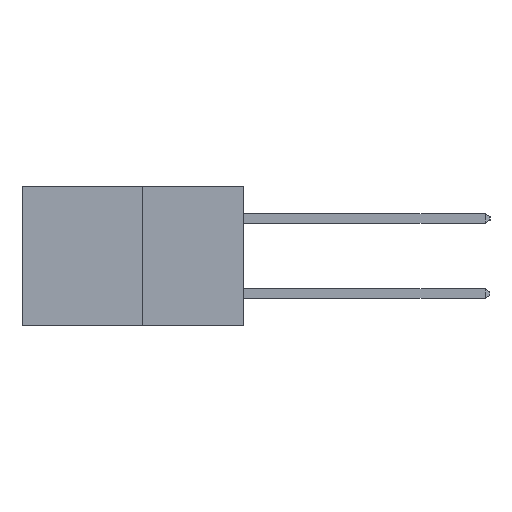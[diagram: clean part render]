
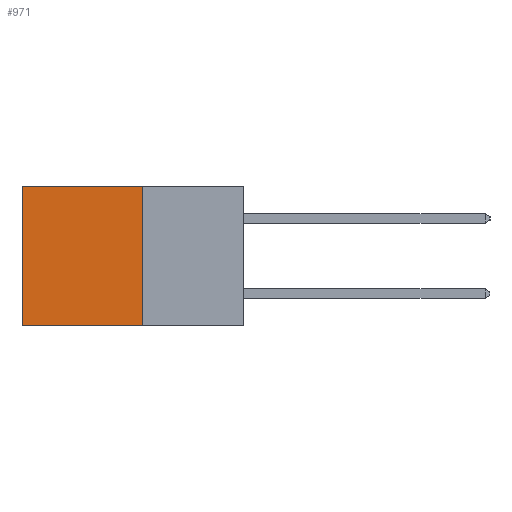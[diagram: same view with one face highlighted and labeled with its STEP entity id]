
A CAD part, left-side view. The second image highlights one B-rep face of the part: STEP entity #971.
In plain terms, the highlighted planar face has unit normal (-1, 0, 0).
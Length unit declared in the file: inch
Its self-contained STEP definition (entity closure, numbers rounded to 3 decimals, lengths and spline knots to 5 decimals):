
#126 = VECTOR ( 'NONE', #10813, 39.37008 ) ;
#417 = CARTESIAN_POINT ( 'NONE',  ( 0.277, 0.59, -0.37 ) ) ;
#971 = ADVANCED_FACE ( 'NONE', ( #7413 ), #9533, .F. ) ;
#1196 = DIRECTION ( 'NONE',  ( 0., 0., -1. ) ) ;
#1204 = VECTOR ( 'NONE', #9394, 39.37008 ) ;
#1546 = CARTESIAN_POINT ( 'NONE',  ( 0.277, 0.59, 0. ) ) ;
#1650 = LINE ( 'NONE', #417, #3403 ) ;
#1742 = LINE ( 'NONE', #2377, #8153 ) ;
#2377 = CARTESIAN_POINT ( 'NONE',  ( 0.277, 0.27, -0.37 ) ) ;
#3048 = CARTESIAN_POINT ( 'NONE',  ( 0.277, 0.27, -0.37 ) ) ;
#3275 = DIRECTION ( 'NONE',  ( 0., 0., -1. ) ) ;
#3356 = VERTEX_POINT ( 'NONE', #1546 ) ;
#3403 = VECTOR ( 'NONE', #4916, 39.37008 ) ;
#4732 = EDGE_CURVE ( 'NONE', #11298, #4774, #10525, .T. ) ;
#4774 = VERTEX_POINT ( 'NONE', #7861 ) ;
#4916 = DIRECTION ( 'NONE',  ( 0., 0., -1. ) ) ;
#4986 = CARTESIAN_POINT ( 'NONE',  ( 0.277, 0.27, -0.37 ) ) ;
#5155 = AXIS2_PLACEMENT_3D ( 'NONE', #4986, #5513, #3275 ) ;
#5362 = CARTESIAN_POINT ( 'NONE',  ( 0.277, 0.27, -0.37 ) ) ;
#5513 = DIRECTION ( 'NONE',  ( 1., 0., 0. ) ) ;
#5731 = VERTEX_POINT ( 'NONE', #8645 ) ;
#5952 = ORIENTED_EDGE ( 'NONE', *, *, #9471, .T. ) ;
#6212 = ORIENTED_EDGE ( 'NONE', *, *, #4732, .F. ) ;
#6231 = EDGE_CURVE ( 'NONE', #5731, #11298, #1742, .T. ) ;
#6398 = CARTESIAN_POINT ( 'NONE',  ( 0.277, 0.27, 0. ) ) ;
#7413 = FACE_OUTER_BOUND ( 'NONE', #7448, .T. ) ;
#7448 = EDGE_LOOP ( 'NONE', ( #5952, #6212, #10013, #9007 ) ) ;
#7861 = CARTESIAN_POINT ( 'NONE',  ( 0.277, 0.59, -0.37 ) ) ;
#8153 = VECTOR ( 'NONE', #1196, 39.37008 ) ;
#8439 = EDGE_CURVE ( 'NONE', #5731, #3356, #9599, .T. ) ;
#8645 = CARTESIAN_POINT ( 'NONE',  ( 0.277, 0.27, 0. ) ) ;
#9007 = ORIENTED_EDGE ( 'NONE', *, *, #8439, .T. ) ;
#9394 = DIRECTION ( 'NONE',  ( 0., 1., 0. ) ) ;
#9471 = EDGE_CURVE ( 'NONE', #3356, #4774, #1650, .T. ) ;
#9533 = PLANE ( 'NONE',  #5155 ) ;
#9599 = LINE ( 'NONE', #6398, #126 ) ;
#10013 = ORIENTED_EDGE ( 'NONE', *, *, #6231, .F. ) ;
#10525 = LINE ( 'NONE', #5362, #1204 ) ;
#10813 = DIRECTION ( 'NONE',  ( 0., 1., 0. ) ) ;
#11298 = VERTEX_POINT ( 'NONE', #3048 ) ;
